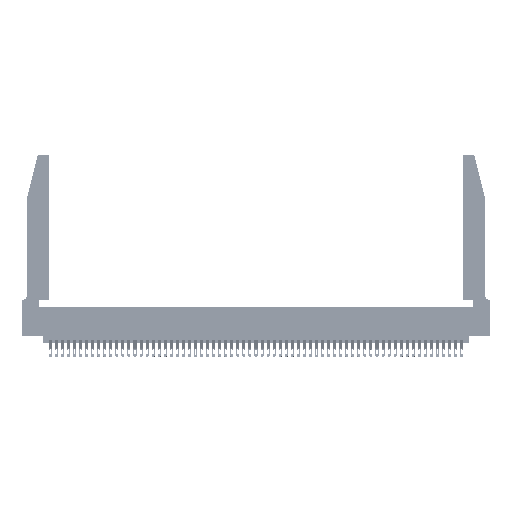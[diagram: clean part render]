
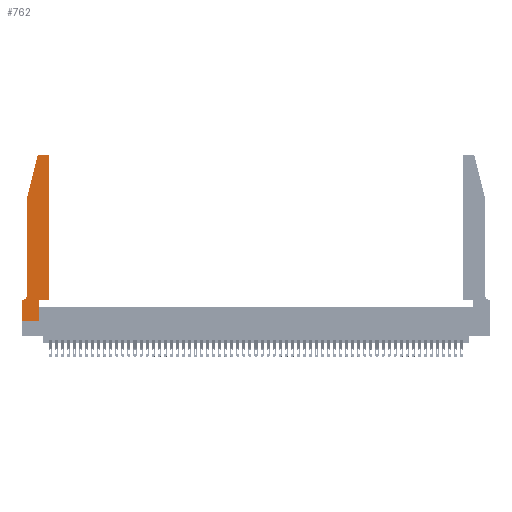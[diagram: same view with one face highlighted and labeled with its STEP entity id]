
A CAD part, top view. The second image highlights one B-rep face of the part: STEP entity #762.
In plain terms, the highlighted planar face has unit normal (0, 0, 1).
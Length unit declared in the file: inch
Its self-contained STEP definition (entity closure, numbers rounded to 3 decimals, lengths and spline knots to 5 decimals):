
#184 = VECTOR ( 'NONE', #3498, 39.37008 ) ;
#762 = ADVANCED_FACE ( 'NONE', ( #52796 ), #1459, .T. ) ;
#992 = CARTESIAN_POINT ( 'NONE',  ( 0.4505, 0.35, 0.37 ) ) ;
#1459 = PLANE ( 'NONE',  #53186 ) ;
#1685 = CARTESIAN_POINT ( 'NONE',  ( 0.0755, 2., 0.37 ) ) ;
#2289 = LINE ( 'NONE', #54056, #2359 ) ;
#2359 = VECTOR ( 'NONE', #46309, 39.37008 ) ;
#3221 = LINE ( 'NONE', #1685, #41594 ) ;
#3498 = DIRECTION ( 'NONE',  ( -1., 0., 0. ) ) ;
#5033 = EDGE_CURVE ( 'NONE', #28125, #51062, #3221, .T. ) ;
#5504 = AXIS2_PLACEMENT_3D ( 'NONE', #26288, #30781, #43548 ) ;
#5648 = LINE ( 'NONE', #36232, #15763 ) ;
#6141 = VERTEX_POINT ( 'NONE', #30493 ) ;
#6301 = CARTESIAN_POINT ( 'NONE',  ( 0.0055, 0.35, 0.37 ) ) ;
#6356 = VERTEX_POINT ( 'NONE', #18780 ) ;
#7626 = VECTOR ( 'NONE', #37354, 39.37008 ) ;
#8140 = VECTOR ( 'NONE', #10162, 39.37008 ) ;
#8616 = AXIS2_PLACEMENT_3D ( 'NONE', #9901, #14260, #22377 ) ;
#8850 = VERTEX_POINT ( 'NONE', #30408 ) ;
#9509 = CARTESIAN_POINT ( 'NONE',  ( 0., 0.35, 0.37 ) ) ;
#9695 = LINE ( 'NONE', #46535, #7626 ) ;
#9769 = CARTESIAN_POINT ( 'NONE',  ( 0.4505, 0.35, 0.37 ) ) ;
#9901 = CARTESIAN_POINT ( 'NONE',  ( 0.4205, 2.72, 0.37 ) ) ;
#9979 = CARTESIAN_POINT ( 'NONE',  ( 0.284, 2.72, 0.37 ) ) ;
#10162 = DIRECTION ( 'NONE',  ( 0., 1., 0. ) ) ;
#10751 = VERTEX_POINT ( 'NONE', #11551 ) ;
#11106 = EDGE_CURVE ( 'NONE', #8850, #39983, #13392, .T. ) ;
#11483 = ORIENTED_EDGE ( 'NONE', *, *, #46840, .T. ) ;
#11551 = CARTESIAN_POINT ( 'NONE',  ( 0., 0.35, 0.37 ) ) ;
#11703 = VECTOR ( 'NONE', #18464, 39.37008 ) ;
#13392 = CIRCLE ( 'NONE', #5504, 0.07 ) ;
#14260 = DIRECTION ( 'NONE',  ( 0., 0., 1. ) ) ;
#14996 = ORIENTED_EDGE ( 'NONE', *, *, #22398, .T. ) ;
#15763 = VECTOR ( 'NONE', #22892, 39.37008 ) ;
#16037 = CIRCLE ( 'NONE', #28075, 0.03 ) ;
#16152 = VECTOR ( 'NONE', #55517, 39.37008 ) ;
#16900 = VERTEX_POINT ( 'NONE', #23255 ) ;
#17442 = VERTEX_POINT ( 'NONE', #48384 ) ;
#18464 = DIRECTION ( 'NONE',  ( 1., 0., 0. ) ) ;
#18700 = DIRECTION ( 'NONE',  ( 0., 1., 0. ) ) ;
#18780 = CARTESIAN_POINT ( 'NONE',  ( 0.2865, 0., 0.37 ) ) ;
#18785 = DIRECTION ( 'NONE',  ( 0., 0., 1. ) ) ;
#19046 = CARTESIAN_POINT ( 'NONE',  ( 0.4505, 2.72, 0.37 ) ) ;
#19987 = EDGE_CURVE ( 'NONE', #16900, #28125, #16037, .T. ) ;
#20091 = CARTESIAN_POINT ( 'NONE',  ( 0.2605, 2.75, 0.37 ) ) ;
#22377 = DIRECTION ( 'NONE',  ( 1., 0., 0. ) ) ;
#22398 = EDGE_CURVE ( 'NONE', #53897, #30009, #44741, .T. ) ;
#22892 = DIRECTION ( 'NONE',  ( 0., -1., 0. ) ) ;
#23255 = CARTESIAN_POINT ( 'NONE',  ( 0.284, 2.75, 0.37 ) ) ;
#23710 = VECTOR ( 'NONE', #18700, 39.37008 ) ;
#24351 = LINE ( 'NONE', #992, #23710 ) ;
#24582 = ORIENTED_EDGE ( 'NONE', *, *, #37187, .T. ) ;
#25706 = LINE ( 'NONE', #36012, #8140 ) ;
#26210 = ORIENTED_EDGE ( 'NONE', *, *, #11106, .T. ) ;
#26288 = CARTESIAN_POINT ( 'NONE',  ( 0.0055, 0.42, 0.37 ) ) ;
#27199 = LINE ( 'NONE', #20091, #184 ) ;
#28075 = AXIS2_PLACEMENT_3D ( 'NONE', #9979, #30732, #43677 ) ;
#28125 = VERTEX_POINT ( 'NONE', #29321 ) ;
#29321 = CARTESIAN_POINT ( 'NONE',  ( 0.25487, 2.72718, 0.37 ) ) ;
#29330 = CARTESIAN_POINT ( 'NONE',  ( 0.4205, 2.75, 0.37 ) ) ;
#30009 = VERTEX_POINT ( 'NONE', #29330 ) ;
#30408 = CARTESIAN_POINT ( 'NONE',  ( 0.0755, 0.42, 0.37 ) ) ;
#30422 = ORIENTED_EDGE ( 'NONE', *, *, #43859, .T. ) ;
#30493 = CARTESIAN_POINT ( 'NONE',  ( 0.4505, 0.35, 0.37 ) ) ;
#30732 = DIRECTION ( 'NONE',  ( 0., 0., 1. ) ) ;
#30781 = DIRECTION ( 'NONE',  ( 0., 0., -1. ) ) ;
#31070 = DIRECTION ( 'NONE',  ( -0.239, -0.971, 0. ) ) ;
#31411 = DIRECTION ( 'NONE',  ( 1., 0., 0. ) ) ;
#31655 = ORIENTED_EDGE ( 'NONE', *, *, #35832, .T. ) ;
#34118 = CARTESIAN_POINT ( 'NONE',  ( 0.2865, 0.35, 0.37 ) ) ;
#35832 = EDGE_CURVE ( 'NONE', #39983, #10751, #2289, .T. ) ;
#36012 = CARTESIAN_POINT ( 'NONE',  ( 0.2865, 0.35, 0.37 ) ) ;
#36232 = CARTESIAN_POINT ( 'NONE',  ( 0.0755, 2., 0.37 ) ) ;
#36235 = EDGE_CURVE ( 'NONE', #44205, #6141, #46063, .T. ) ;
#37187 = EDGE_CURVE ( 'NONE', #30009, #16900, #27199, .T. ) ;
#37354 = DIRECTION ( 'NONE',  ( 1., 0., 0. ) ) ;
#37668 = ORIENTED_EDGE ( 'NONE', *, *, #55422, .T. ) ;
#37890 = ORIENTED_EDGE ( 'NONE', *, *, #19987, .T. ) ;
#38210 = ORIENTED_EDGE ( 'NONE', *, *, #5033, .T. ) ;
#39550 = ORIENTED_EDGE ( 'NONE', *, *, #53760, .T. ) ;
#39602 = ORIENTED_EDGE ( 'NONE', *, *, #36235, .T. ) ;
#39983 = VERTEX_POINT ( 'NONE', #6301 ) ;
#41594 = VECTOR ( 'NONE', #31070, 39.37008 ) ;
#43056 = CARTESIAN_POINT ( 'NONE',  ( 0., 0., 0.37 ) ) ;
#43548 = DIRECTION ( 'NONE',  ( -1., 0., 0. ) ) ;
#43647 = LINE ( 'NONE', #43056, #16152 ) ;
#43677 = DIRECTION ( 'NONE',  ( 1., 0., 0. ) ) ;
#43859 = EDGE_CURVE ( 'NONE', #51062, #8850, #5648, .T. ) ;
#44035 = EDGE_LOOP ( 'NONE', ( #24582, #37890, #38210, #30422, #26210, #31655, #37668, #11483, #44238, #39602, #39550, #14996 ) ) ;
#44205 = VERTEX_POINT ( 'NONE', #34118 ) ;
#44238 = ORIENTED_EDGE ( 'NONE', *, *, #53937, .T. ) ;
#44741 = CIRCLE ( 'NONE', #8616, 0.03 ) ;
#46063 = LINE ( 'NONE', #9769, #11703 ) ;
#46309 = DIRECTION ( 'NONE',  ( -1., 0., 0. ) ) ;
#46535 = CARTESIAN_POINT ( 'NONE',  ( 0., 0., 0.37 ) ) ;
#46840 = EDGE_CURVE ( 'NONE', #17442, #6356, #9695, .T. ) ;
#48384 = CARTESIAN_POINT ( 'NONE',  ( 0., 0., 0.37 ) ) ;
#49074 = CARTESIAN_POINT ( 'NONE',  ( 0.0755, 2., 0.37 ) ) ;
#51062 = VERTEX_POINT ( 'NONE', #49074 ) ;
#52796 = FACE_OUTER_BOUND ( 'NONE', #44035, .T. ) ;
#53186 = AXIS2_PLACEMENT_3D ( 'NONE', #9509, #18785, #31411 ) ;
#53760 = EDGE_CURVE ( 'NONE', #6141, #53897, #24351, .T. ) ;
#53897 = VERTEX_POINT ( 'NONE', #19046 ) ;
#53937 = EDGE_CURVE ( 'NONE', #6356, #44205, #25706, .T. ) ;
#54056 = CARTESIAN_POINT ( 'NONE',  ( 0.0755, 0.35, 0.37 ) ) ;
#55422 = EDGE_CURVE ( 'NONE', #10751, #17442, #43647, .T. ) ;
#55517 = DIRECTION ( 'NONE',  ( 0., -1., 0. ) ) ;
